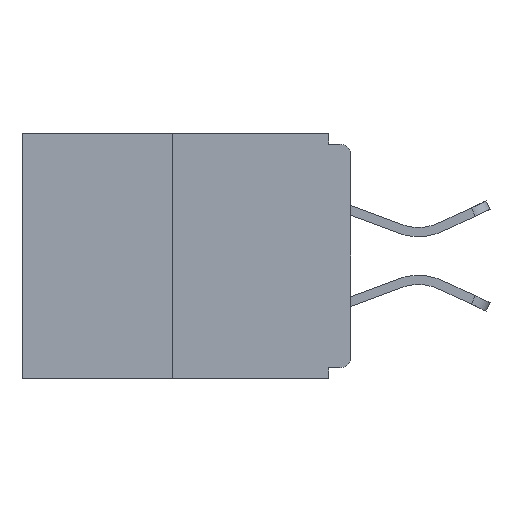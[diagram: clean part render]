
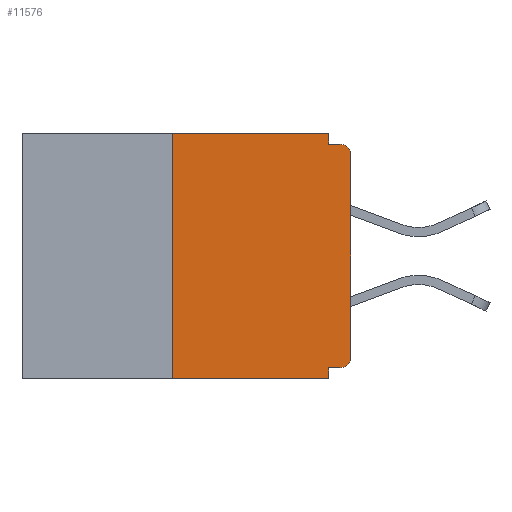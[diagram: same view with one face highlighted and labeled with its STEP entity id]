
A CAD part, left-side view. The second image highlights one B-rep face of the part: STEP entity #11576.
In plain terms, the highlighted planar face has unit normal (-1, 0, 0).
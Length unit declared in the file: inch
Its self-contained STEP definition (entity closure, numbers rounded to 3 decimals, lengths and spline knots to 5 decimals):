
#53 = LINE ( 'NONE', #22145, #2735 ) ;
#886 = DIRECTION ( 'NONE',  ( 1., 0., 0. ) ) ;
#1302 = LINE ( 'NONE', #11233, #21039 ) ;
#1565 = VERTEX_POINT ( 'NONE', #2331 ) ;
#2048 = EDGE_CURVE ( 'NONE', #19555, #20964, #15267, .T. ) ;
#2331 = CARTESIAN_POINT ( 'NONE',  ( 0., 0.031, -0.015 ) ) ;
#2581 = VECTOR ( 'NONE', #14180, 39.37008 ) ;
#2598 = CARTESIAN_POINT ( 'NONE',  ( 0., 0.031, 0. ) ) ;
#2735 = VECTOR ( 'NONE', #23683, 39.37008 ) ;
#2763 = EDGE_CURVE ( 'NONE', #20964, #14399, #22746, .T. ) ;
#3223 = CARTESIAN_POINT ( 'NONE',  ( 0., 0., -0.328 ) ) ;
#3268 = ORIENTED_EDGE ( 'NONE', *, *, #18915, .F. ) ;
#3465 = DIRECTION ( 'NONE',  ( -1., 0., 0. ) ) ;
#3551 = CARTESIAN_POINT ( 'NONE',  ( 0., 0.031, -0.328 ) ) ;
#3686 = EDGE_CURVE ( 'NONE', #4904, #12806, #5275, .T. ) ;
#4057 = VERTEX_POINT ( 'NONE', #15140 ) ;
#4135 = DIRECTION ( 'NONE',  ( 0., 0., -1. ) ) ;
#4540 = CARTESIAN_POINT ( 'NONE',  ( 0., 0., -0.03 ) ) ;
#4541 = EDGE_CURVE ( 'NONE', #20187, #1565, #20490, .T. ) ;
#4904 = VERTEX_POINT ( 'NONE', #3551 ) ;
#5275 = LINE ( 'NONE', #15655, #5901 ) ;
#5442 = VECTOR ( 'NONE', #15172, 39.37008 ) ;
#5646 = EDGE_CURVE ( 'NONE', #16545, #4904, #7304, .T. ) ;
#5901 = VECTOR ( 'NONE', #4135, 39.37008 ) ;
#5980 = ORIENTED_EDGE ( 'NONE', *, *, #19060, .F. ) ;
#6608 = VECTOR ( 'NONE', #20873, 39.37008 ) ;
#6982 = ORIENTED_EDGE ( 'NONE', *, *, #4541, .F. ) ;
#7304 = LINE ( 'NONE', #3223, #16257 ) ;
#9774 = VERTEX_POINT ( 'NONE', #11697 ) ;
#10380 = CARTESIAN_POINT ( 'NONE',  ( 0., 0.46, -0.343 ) ) ;
#10578 = DIRECTION ( 'NONE',  ( 0., 0., -1. ) ) ;
#11107 = LINE ( 'NONE', #15424, #5442 ) ;
#11233 = CARTESIAN_POINT ( 'NONE',  ( 0., 0., -0.015 ) ) ;
#11261 = CARTESIAN_POINT ( 'NONE',  ( 0., 0.015, -0.328 ) ) ;
#11576 = ADVANCED_FACE ( 'NONE', ( #11744 ), #22102, .F. ) ;
#11697 = CARTESIAN_POINT ( 'NONE',  ( 0., 0.25, -0.343 ) ) ;
#11744 = FACE_OUTER_BOUND ( 'NONE', #20508, .T. ) ;
#11923 = CARTESIAN_POINT ( 'NONE',  ( 0., 0.031, 0. ) ) ;
#12243 = DIRECTION ( 'NONE',  ( -1., 0., 0. ) ) ;
#12519 = DIRECTION ( 'NONE',  ( 0., -1., 0. ) ) ;
#12806 = VERTEX_POINT ( 'NONE', #15898 ) ;
#12885 = CARTESIAN_POINT ( 'NONE',  ( 0., 0.015, -0.03 ) ) ;
#13161 = DIRECTION ( 'NONE',  ( 0., -1., 0. ) ) ;
#14180 = DIRECTION ( 'NONE',  ( 0., 0., -1. ) ) ;
#14215 = CARTESIAN_POINT ( 'NONE',  ( 0., 0.46, 0. ) ) ;
#14399 = VERTEX_POINT ( 'NONE', #16800 ) ;
#14852 = VECTOR ( 'NONE', #12519, 39.37008 ) ;
#15140 = CARTESIAN_POINT ( 'NONE',  ( 0., 0.25, 0. ) ) ;
#15172 = DIRECTION ( 'NONE',  ( 0., 0., 1. ) ) ;
#15267 = LINE ( 'NONE', #15776, #6608 ) ;
#15424 = CARTESIAN_POINT ( 'NONE',  ( 0., 0.25, 0. ) ) ;
#15655 = CARTESIAN_POINT ( 'NONE',  ( 0., 0.031, -0.343 ) ) ;
#15776 = CARTESIAN_POINT ( 'NONE',  ( 0., 0., 0. ) ) ;
#15898 = CARTESIAN_POINT ( 'NONE',  ( 0., 0.031, -0.343 ) ) ;
#15929 = ORIENTED_EDGE ( 'NONE', *, *, #2048, .T. ) ;
#16241 = EDGE_CURVE ( 'NONE', #9774, #12806, #16651, .T. ) ;
#16257 = VECTOR ( 'NONE', #16393, 39.37008 ) ;
#16393 = DIRECTION ( 'NONE',  ( 0., 1., 0. ) ) ;
#16545 = VERTEX_POINT ( 'NONE', #11261 ) ;
#16651 = LINE ( 'NONE', #10380, #14852 ) ;
#16800 = CARTESIAN_POINT ( 'NONE',  ( 0., 0.015, -0.015 ) ) ;
#17502 = ORIENTED_EDGE ( 'NONE', *, *, #19838, .F. ) ;
#17949 = AXIS2_PLACEMENT_3D ( 'NONE', #12885, #3465, #20679 ) ;
#18528 = AXIS2_PLACEMENT_3D ( 'NONE', #20192, #12243, #10578 ) ;
#18637 = CARTESIAN_POINT ( 'NONE',  ( 0., 0., -0.313 ) ) ;
#18915 = EDGE_CURVE ( 'NONE', #1565, #14399, #1302, .T. ) ;
#19060 = EDGE_CURVE ( 'NONE', #9774, #4057, #11107, .T. ) ;
#19555 = VERTEX_POINT ( 'NONE', #18637 ) ;
#19838 = EDGE_CURVE ( 'NONE', #4057, #20187, #53, .T. ) ;
#20187 = VERTEX_POINT ( 'NONE', #11923 ) ;
#20192 = CARTESIAN_POINT ( 'NONE',  ( 0., 0.015, -0.313 ) ) ;
#20408 = EDGE_CURVE ( 'NONE', #16545, #19555, #24254, .T. ) ;
#20490 = LINE ( 'NONE', #2598, #2581 ) ;
#20508 = EDGE_LOOP ( 'NONE', ( #17502, #5980, #20515, #21097, #20954, #23394, #15929, #23023, #3268, #6982 ) ) ;
#20515 = ORIENTED_EDGE ( 'NONE', *, *, #16241, .T. ) ;
#20679 = DIRECTION ( 'NONE',  ( 0., 0., -1. ) ) ;
#20873 = DIRECTION ( 'NONE',  ( 0., 0., 1. ) ) ;
#20954 = ORIENTED_EDGE ( 'NONE', *, *, #5646, .F. ) ;
#20964 = VERTEX_POINT ( 'NONE', #4540 ) ;
#21039 = VECTOR ( 'NONE', #13161, 39.37008 ) ;
#21097 = ORIENTED_EDGE ( 'NONE', *, *, #3686, .F. ) ;
#21321 = AXIS2_PLACEMENT_3D ( 'NONE', #14215, #886, #23804 ) ;
#22102 = PLANE ( 'NONE',  #21321 ) ;
#22145 = CARTESIAN_POINT ( 'NONE',  ( 0., 0.46, 0. ) ) ;
#22746 = CIRCLE ( 'NONE', #17949, 0.015 ) ;
#23023 = ORIENTED_EDGE ( 'NONE', *, *, #2763, .T. ) ;
#23394 = ORIENTED_EDGE ( 'NONE', *, *, #20408, .T. ) ;
#23683 = DIRECTION ( 'NONE',  ( 0., -1., 0. ) ) ;
#23804 = DIRECTION ( 'NONE',  ( 0., 0., -1. ) ) ;
#24254 = CIRCLE ( 'NONE', #18528, 0.015 ) ;
